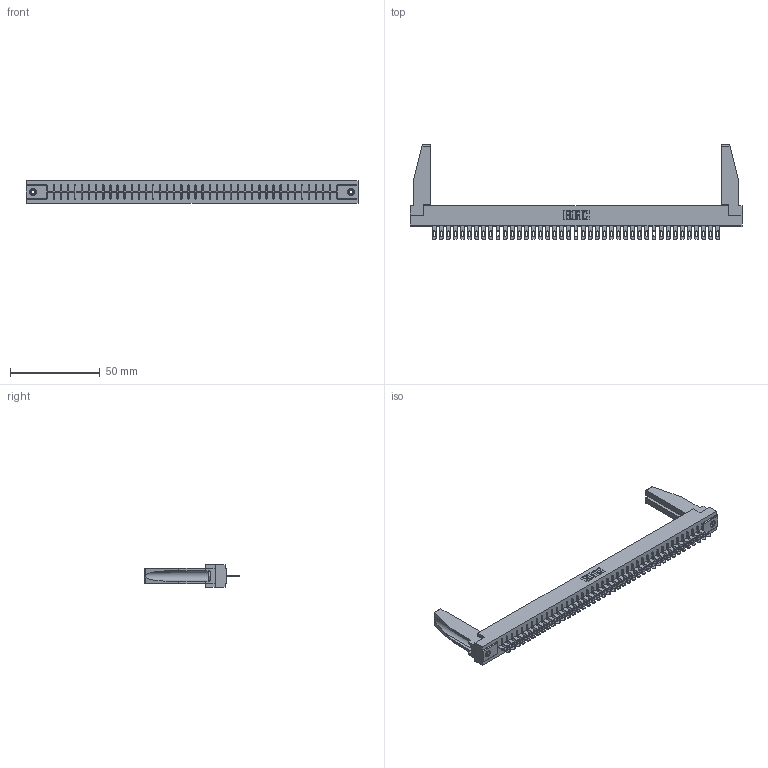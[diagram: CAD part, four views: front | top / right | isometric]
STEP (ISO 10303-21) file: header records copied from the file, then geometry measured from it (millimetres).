
FILE_DESCRIPTION (( 'STEP AP203' ), '1' );
FILE_NAME ('316-041-400-178.STEP', '2020-09-23T07:03:22', ( '' ), ( '' ), 'SwSTEP 2.0', 'SolidWorks 2020', '' );
FILE_SCHEMA (( 'CONFIG_CONTROL_DESIGN' ));
Length unit declared in the file: inch
Products named in the file (5): 306-290-001_100; 316-041-400-178; 307-220-078; 306 Part_.156 Dia; 345-250-001_345-250-001-102
Assembly tree (46 placements, depth 2):
  316-041-400-178
    306 Part_.156 Dia
    306-290-001_100  x41
    345-250-001_345-250-001-102  x2
    307-220-078  x2
Bounding box: 185.47 x 52.91 x 12.7 mm (x, y, z)
Volume: 24635.1 mm3; surface area: 25716.1 mm2
Topology: 46 solids, 46 shells, 3362 faces, 9461 edges, 6078 vertices
Faces by surface type: plane 2202, cylinder 980, sphere 164, cone 12, torus 4
Entity records: 40967 total; most frequent: CARTESIAN_POINT 6880, ORIENTED_EDGE 6780, DIRECTION 6736, EDGE_CURVE 3390, LINE 2652, VECTOR 2652, VERTEX_POINT 2144, AXIS2_PLACEMENT_3D 2042
